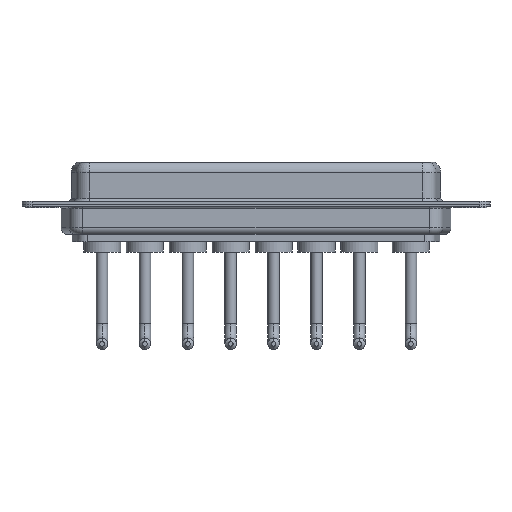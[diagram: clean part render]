
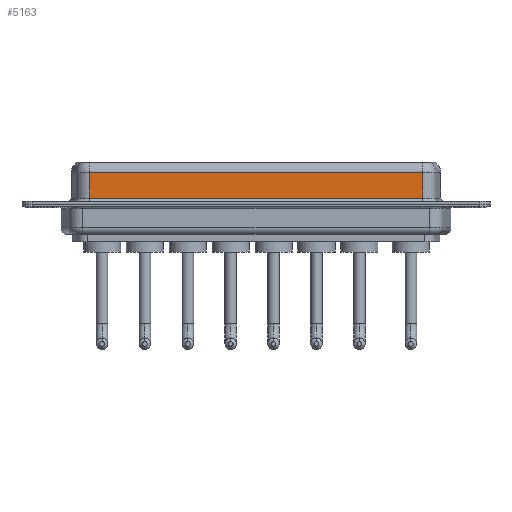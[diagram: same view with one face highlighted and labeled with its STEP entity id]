
A CAD part, front view. The second image highlights one B-rep face of the part: STEP entity #5163.
In plain terms, the highlighted planar face has unit normal (0, -1, 0).
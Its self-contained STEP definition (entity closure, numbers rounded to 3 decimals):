
#194 = EDGE_CURVE ( 'NONE', #1811, #10977, #5108, .T. ) ;
#262 = EDGE_LOOP ( 'NONE', ( #6858, #11020, #3242, #1812 ) ) ;
#494 = CARTESIAN_POINT ( 'NONE',  ( 56.462, -3.95, 0.9 ) ) ;
#520 = VERTEX_POINT ( 'NONE', #9945 ) ;
#648 = CARTESIAN_POINT ( 'NONE',  ( 56.462, -3.95, 4.65 ) ) ;
#1772 = DIRECTION ( 'NONE',  ( 0., 1., 0. ) ) ;
#1811 = VERTEX_POINT ( 'NONE', #8542 ) ;
#1812 = ORIENTED_EDGE ( 'NONE', *, *, #9195, .T. ) ;
#1868 = AXIS2_PLACEMENT_3D ( 'NONE', #4490, #1772, #10620 ) ;
#2132 = LINE ( 'NONE', #494, #4021 ) ;
#2754 = PLANE ( 'NONE',  #1868 ) ;
#3241 = DIRECTION ( 'NONE',  ( 0., 0., -1. ) ) ;
#3242 = ORIENTED_EDGE ( 'NONE', *, *, #5549, .T. ) ;
#3318 = DIRECTION ( 'NONE',  ( -1., 0., 0. ) ) ;
#3353 = VECTOR ( 'NONE', #3318, 1000. ) ;
#4021 = VECTOR ( 'NONE', #6692, 1000. ) ;
#4309 = LINE ( 'NONE', #5335, #9477 ) ;
#4377 = FACE_OUTER_BOUND ( 'NONE', #262, .T. ) ;
#4490 = CARTESIAN_POINT ( 'NONE',  ( 56.462, -3.95, 6.4 ) ) ;
#5099 = DIRECTION ( 'NONE',  ( 0., 0., -1. ) ) ;
#5108 = LINE ( 'NONE', #648, #3353 ) ;
#5163 = ADVANCED_FACE ( 'NONE', ( #4377 ), #2754, .F. ) ;
#5299 = VECTOR ( 'NONE', #3241, 1000. ) ;
#5335 = CARTESIAN_POINT ( 'NONE',  ( 7.038, -3.95, 6.4 ) ) ;
#5549 = EDGE_CURVE ( 'NONE', #10977, #8735, #4309, .T. ) ;
#6692 = DIRECTION ( 'NONE',  ( 1., 0., 0. ) ) ;
#6858 = ORIENTED_EDGE ( 'NONE', *, *, #7135, .F. ) ;
#7135 = EDGE_CURVE ( 'NONE', #1811, #520, #10297, .T. ) ;
#7261 = CARTESIAN_POINT ( 'NONE',  ( 7.038, -3.95, 0.9 ) ) ;
#8542 = CARTESIAN_POINT ( 'NONE',  ( 56.462, -3.95, 4.65 ) ) ;
#8735 = VERTEX_POINT ( 'NONE', #7261 ) ;
#8827 = CARTESIAN_POINT ( 'NONE',  ( 7.038, -3.95, 4.65 ) ) ;
#9195 = EDGE_CURVE ( 'NONE', #8735, #520, #2132, .T. ) ;
#9477 = VECTOR ( 'NONE', #5099, 1000. ) ;
#9945 = CARTESIAN_POINT ( 'NONE',  ( 56.462, -3.95, 0.9 ) ) ;
#9955 = CARTESIAN_POINT ( 'NONE',  ( 56.462, -3.95, 6.4 ) ) ;
#10297 = LINE ( 'NONE', #9955, #5299 ) ;
#10620 = DIRECTION ( 'NONE',  ( 0., 0., 1. ) ) ;
#10977 = VERTEX_POINT ( 'NONE', #8827 ) ;
#11020 = ORIENTED_EDGE ( 'NONE', *, *, #194, .T. ) ;
